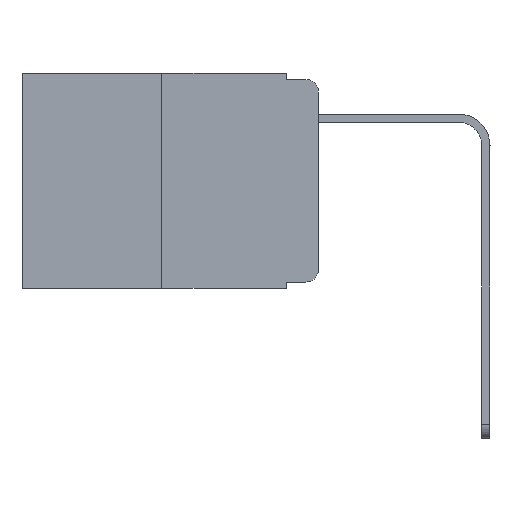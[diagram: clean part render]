
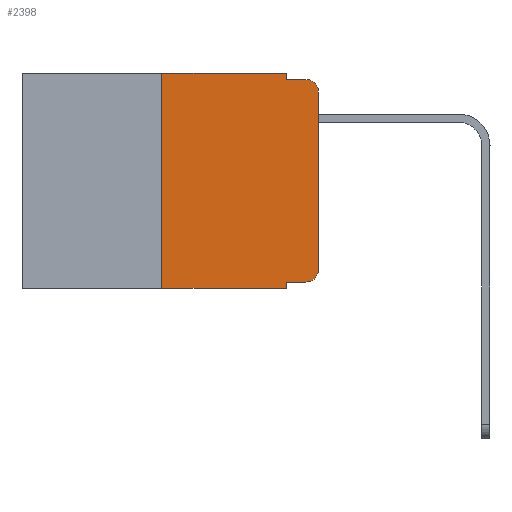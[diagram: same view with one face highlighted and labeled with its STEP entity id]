
A CAD part, left-side view. The second image highlights one B-rep face of the part: STEP entity #2398.
In plain terms, the highlighted planar face has unit normal (-1, 0, 0).
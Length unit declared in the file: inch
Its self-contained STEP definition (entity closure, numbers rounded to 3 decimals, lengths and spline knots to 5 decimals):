
#114 = DIRECTION ( 'NONE',  ( 0., 0., -1. ) ) ;
#230 = CIRCLE ( 'NONE', #12670, 0.02 ) ;
#421 = VECTOR ( 'NONE', #2789, 39.37008 ) ;
#476 = CARTESIAN_POINT ( 'NONE',  ( 0., 0.25, -0.343 ) ) ;
#572 = VERTEX_POINT ( 'NONE', #9536 ) ;
#1446 = EDGE_CURVE ( 'NONE', #14735, #18943, #16152, .T. ) ;
#1716 = CARTESIAN_POINT ( 'NONE',  ( 0., 0.25, 0. ) ) ;
#1824 = ORIENTED_EDGE ( 'NONE', *, *, #1446, .F. ) ;
#2077 = VERTEX_POINT ( 'NONE', #9798 ) ;
#2156 = CARTESIAN_POINT ( 'NONE',  ( 0., 0.051, 0. ) ) ;
#2289 = ORIENTED_EDGE ( 'NONE', *, *, #14240, .T. ) ;
#2398 = ADVANCED_FACE ( 'NONE', ( #16117 ), #6252, .F. ) ;
#2519 = DIRECTION ( 'NONE',  ( 0., 0., 1. ) ) ;
#2522 = CARTESIAN_POINT ( 'NONE',  ( 0., 0.051, 0. ) ) ;
#2789 = DIRECTION ( 'NONE',  ( 0., -1., 0. ) ) ;
#3289 = VERTEX_POINT ( 'NONE', #1716 ) ;
#3529 = DIRECTION ( 'NONE',  ( 0., 0., -1. ) ) ;
#3571 = ORIENTED_EDGE ( 'NONE', *, *, #12032, .T. ) ;
#4141 = CARTESIAN_POINT ( 'NONE',  ( 0., 0.473, -0.343 ) ) ;
#4515 = DIRECTION ( 'NONE',  ( 1., 0., 0. ) ) ;
#5012 = LINE ( 'NONE', #6743, #12104 ) ;
#5328 = CARTESIAN_POINT ( 'NONE',  ( 0., 0., -0.313 ) ) ;
#6252 = PLANE ( 'NONE',  #14574 ) ;
#6260 = LINE ( 'NONE', #2522, #17943 ) ;
#6300 = EDGE_CURVE ( 'NONE', #12097, #3289, #5012, .T. ) ;
#6350 = DIRECTION ( 'NONE',  ( 0., -1., 0. ) ) ;
#6431 = CARTESIAN_POINT ( 'NONE',  ( 0., 0.02, -0.03 ) ) ;
#6522 = EDGE_LOOP ( 'NONE', ( #10490, #17664, #17923, #1824, #17585, #9665, #2289, #11413, #3571, #14077 ) ) ;
#6743 = CARTESIAN_POINT ( 'NONE',  ( 0., 0.25, 0. ) ) ;
#6960 = VECTOR ( 'NONE', #10646, 39.37008 ) ;
#6985 = CARTESIAN_POINT ( 'NONE',  ( 0., 0.051, -0.343 ) ) ;
#7081 = EDGE_CURVE ( 'NONE', #17550, #572, #11619, .T. ) ;
#7424 = CARTESIAN_POINT ( 'NONE',  ( 0., 0.02, -0.333 ) ) ;
#7581 = AXIS2_PLACEMENT_3D ( 'NONE', #6431, #18139, #3529 ) ;
#7704 = CARTESIAN_POINT ( 'NONE',  ( 0., 0.051, -0.333 ) ) ;
#8897 = CARTESIAN_POINT ( 'NONE',  ( 0., 0.473, 0. ) ) ;
#9536 = CARTESIAN_POINT ( 'NONE',  ( 0., 0., -0.03 ) ) ;
#9665 = ORIENTED_EDGE ( 'NONE', *, *, #6300, .F. ) ;
#9798 = CARTESIAN_POINT ( 'NONE',  ( 0., 0.051, -0.333 ) ) ;
#9865 = EDGE_CURVE ( 'NONE', #2077, #18597, #6260, .T. ) ;
#10254 = EDGE_CURVE ( 'NONE', #3289, #14735, #14491, .T. ) ;
#10490 = ORIENTED_EDGE ( 'NONE', *, *, #7081, .T. ) ;
#10646 = DIRECTION ( 'NONE',  ( 0., -1., 0. ) ) ;
#10709 = CARTESIAN_POINT ( 'NONE',  ( 0., 0.473, 0. ) ) ;
#11413 = ORIENTED_EDGE ( 'NONE', *, *, #9865, .F. ) ;
#11619 = LINE ( 'NONE', #14296, #18261 ) ;
#11761 = CIRCLE ( 'NONE', #7581, 0.02 ) ;
#12032 = EDGE_CURVE ( 'NONE', #2077, #15974, #14472, .T. ) ;
#12097 = VERTEX_POINT ( 'NONE', #476 ) ;
#12104 = VECTOR ( 'NONE', #15658, 39.37008 ) ;
#12217 = DIRECTION ( 'NONE',  ( -1., 0., 0. ) ) ;
#12394 = DIRECTION ( 'NONE',  ( 0., 0., -1. ) ) ;
#12599 = CARTESIAN_POINT ( 'NONE',  ( 0., 0.051, -0.01 ) ) ;
#12667 = VECTOR ( 'NONE', #6350, 39.37008 ) ;
#12670 = AXIS2_PLACEMENT_3D ( 'NONE', #13959, #12217, #16915 ) ;
#12756 = CARTESIAN_POINT ( 'NONE',  ( 0., 0.051, 0. ) ) ;
#13153 = CARTESIAN_POINT ( 'NONE',  ( 0., 0.02, -0.01 ) ) ;
#13322 = EDGE_CURVE ( 'NONE', #15974, #17550, #230, .T. ) ;
#13951 = LINE ( 'NONE', #4141, #421 ) ;
#13959 = CARTESIAN_POINT ( 'NONE',  ( 0., 0.02, -0.313 ) ) ;
#14077 = ORIENTED_EDGE ( 'NONE', *, *, #13322, .T. ) ;
#14081 = DIRECTION ( 'NONE',  ( 0., -1., 0. ) ) ;
#14131 = VECTOR ( 'NONE', #12394, 39.37008 ) ;
#14179 = DIRECTION ( 'NONE',  ( 0., 0., -1. ) ) ;
#14240 = EDGE_CURVE ( 'NONE', #12097, #18597, #13951, .T. ) ;
#14296 = CARTESIAN_POINT ( 'NONE',  ( 0., 0., 0. ) ) ;
#14472 = LINE ( 'NONE', #7704, #6960 ) ;
#14491 = LINE ( 'NONE', #10709, #12667 ) ;
#14574 = AXIS2_PLACEMENT_3D ( 'NONE', #8897, #4515, #114 ) ;
#14735 = VERTEX_POINT ( 'NONE', #12756 ) ;
#15658 = DIRECTION ( 'NONE',  ( 0., 0., 1. ) ) ;
#15897 = VERTEX_POINT ( 'NONE', #13153 ) ;
#15974 = VERTEX_POINT ( 'NONE', #7424 ) ;
#16117 = FACE_OUTER_BOUND ( 'NONE', #6522, .T. ) ;
#16152 = LINE ( 'NONE', #2156, #14131 ) ;
#16593 = CARTESIAN_POINT ( 'NONE',  ( 0., 0.051, -0.01 ) ) ;
#16915 = DIRECTION ( 'NONE',  ( 0., 0., -1. ) ) ;
#16971 = EDGE_CURVE ( 'NONE', #572, #15897, #11761, .T. ) ;
#17216 = LINE ( 'NONE', #12599, #18352 ) ;
#17550 = VERTEX_POINT ( 'NONE', #5328 ) ;
#17585 = ORIENTED_EDGE ( 'NONE', *, *, #10254, .F. ) ;
#17607 = EDGE_CURVE ( 'NONE', #18943, #15897, #17216, .T. ) ;
#17664 = ORIENTED_EDGE ( 'NONE', *, *, #16971, .T. ) ;
#17923 = ORIENTED_EDGE ( 'NONE', *, *, #17607, .F. ) ;
#17943 = VECTOR ( 'NONE', #14179, 39.37008 ) ;
#18139 = DIRECTION ( 'NONE',  ( -1., 0., 0. ) ) ;
#18261 = VECTOR ( 'NONE', #2519, 39.37008 ) ;
#18352 = VECTOR ( 'NONE', #14081, 39.37008 ) ;
#18597 = VERTEX_POINT ( 'NONE', #6985 ) ;
#18943 = VERTEX_POINT ( 'NONE', #16593 ) ;
